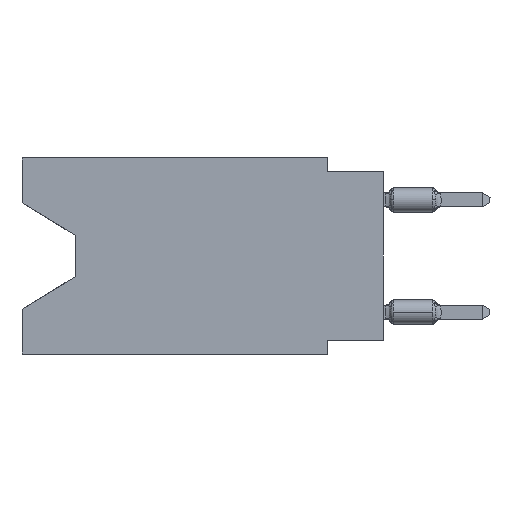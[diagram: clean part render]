
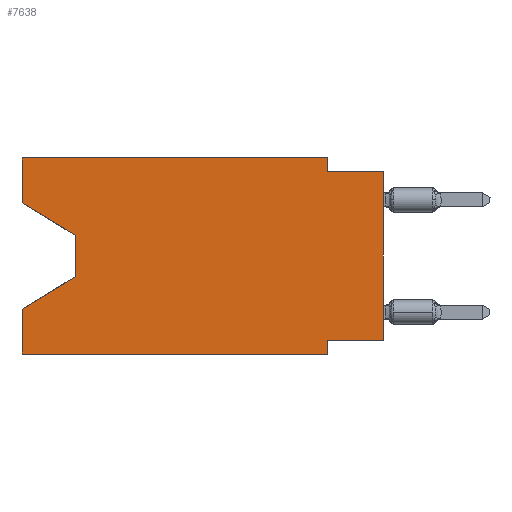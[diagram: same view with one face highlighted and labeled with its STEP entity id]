
A CAD part, left-side view. The second image highlights one B-rep face of the part: STEP entity #7638.
In plain terms, the highlighted planar face has unit normal (-1, 0, 0).
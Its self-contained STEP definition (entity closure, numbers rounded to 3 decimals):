
#333 = VECTOR ( 'NONE', #24219, 1000. ) ;
#567 = CARTESIAN_POINT ( 'NONE',  ( 0., 16.383, 0. ) ) ;
#601 = CARTESIAN_POINT ( 'NONE',  ( 0., 13.97, -5.385 ) ) ;
#702 = EDGE_CURVE ( 'NONE', #13876, #2454, #21498, .T. ) ;
#1024 = DIRECTION ( 'NONE',  ( 0., -1., 0. ) ) ;
#1044 = VECTOR ( 'NONE', #23749, 1000. ) ;
#1051 = CARTESIAN_POINT ( 'NONE',  ( 0., 16.383, 0. ) ) ;
#1136 = VECTOR ( 'NONE', #9603, 1000. ) ;
#1296 = VECTOR ( 'NONE', #15050, 1000. ) ;
#1582 = EDGE_LOOP ( 'NONE', ( #3260, #3955, #20768, #3757, #7621, #11592, #12425, #11807, #28553, #17022, #10541, #20219 ) ) ;
#2454 = VERTEX_POINT ( 'NONE', #13419 ) ;
#2486 = VECTOR ( 'NONE', #19190, 1000. ) ;
#2533 = EDGE_CURVE ( 'NONE', #17862, #22297, #10644, .T. ) ;
#2642 = VECTOR ( 'NONE', #14974, 1000. ) ;
#3260 = ORIENTED_EDGE ( 'NONE', *, *, #9465, .T. ) ;
#3692 = EDGE_CURVE ( 'NONE', #17862, #13538, #23213, .T. ) ;
#3741 = VECTOR ( 'NONE', #12759, 1000. ) ;
#3757 = ORIENTED_EDGE ( 'NONE', *, *, #12318, .F. ) ;
#3955 = ORIENTED_EDGE ( 'NONE', *, *, #20368, .T. ) ;
#4307 = EDGE_CURVE ( 'NONE', #2454, #22297, #23938, .T. ) ;
#4507 = LINE ( 'NONE', #23024, #11135 ) ;
#4675 = CARTESIAN_POINT ( 'NONE',  ( 0., 0., -8.255 ) ) ;
#4863 = VERTEX_POINT ( 'NONE', #23755 ) ;
#5017 = LINE ( 'NONE', #16282, #16054 ) ;
#5387 = VERTEX_POINT ( 'NONE', #29413 ) ;
#5941 = CARTESIAN_POINT ( 'NONE',  ( 0., 16.383, 0. ) ) ;
#7077 = LINE ( 'NONE', #12732, #1296 ) ;
#7621 = ORIENTED_EDGE ( 'NONE', *, *, #10113, .T. ) ;
#7638 = ADVANCED_FACE ( 'NONE', ( #10251 ), #17053, .F. ) ;
#8627 = VECTOR ( 'NONE', #15701, 1000. ) ;
#9268 = DIRECTION ( 'NONE',  ( 0., -0.855, -0.519 ) ) ;
#9465 = EDGE_CURVE ( 'NONE', #11706, #21772, #4507, .T. ) ;
#9603 = DIRECTION ( 'NONE',  ( 0., 1., 0. ) ) ;
#9775 = CARTESIAN_POINT ( 'NONE',  ( 0., 2.54, 0. ) ) ;
#10103 = DIRECTION ( 'NONE',  ( 1., 0., 0. ) ) ;
#10113 = EDGE_CURVE ( 'NONE', #15246, #10307, #7077, .T. ) ;
#10115 = CARTESIAN_POINT ( 'NONE',  ( 0., 2.54, 0. ) ) ;
#10251 = FACE_OUTER_BOUND ( 'NONE', #1582, .T. ) ;
#10307 = VERTEX_POINT ( 'NONE', #27705 ) ;
#10541 = ORIENTED_EDGE ( 'NONE', *, *, #26278, .F. ) ;
#10644 = LINE ( 'NONE', #17600, #13380 ) ;
#11135 = VECTOR ( 'NONE', #9268, 1000. ) ;
#11202 = EDGE_CURVE ( 'NONE', #11706, #5387, #24356, .T. ) ;
#11592 = ORIENTED_EDGE ( 'NONE', *, *, #20954, .F. ) ;
#11706 = VERTEX_POINT ( 'NONE', #29972 ) ;
#11807 = ORIENTED_EDGE ( 'NONE', *, *, #2533, .T. ) ;
#12318 = EDGE_CURVE ( 'NONE', #15246, #27703, #26377, .T. ) ;
#12425 = ORIENTED_EDGE ( 'NONE', *, *, #3692, .F. ) ;
#12732 = CARTESIAN_POINT ( 'NONE',  ( 0., 16.383, -8.89 ) ) ;
#12759 = DIRECTION ( 'NONE',  ( 0., 0., 1. ) ) ;
#13380 = VECTOR ( 'NONE', #27020, 1000. ) ;
#13419 = CARTESIAN_POINT ( 'NONE',  ( 0., 2.54, -0.635 ) ) ;
#13538 = VERTEX_POINT ( 'NONE', #24063 ) ;
#13876 = VERTEX_POINT ( 'NONE', #10115 ) ;
#14329 = CARTESIAN_POINT ( 'NONE',  ( 0., 16.383, 0. ) ) ;
#14974 = DIRECTION ( 'NONE',  ( 0., -1., 0. ) ) ;
#15050 = DIRECTION ( 'NONE',  ( 0., -1., 0. ) ) ;
#15246 = VERTEX_POINT ( 'NONE', #22180 ) ;
#15701 = DIRECTION ( 'NONE',  ( 0., 0., -1. ) ) ;
#16007 = LINE ( 'NONE', #20189, #8627 ) ;
#16054 = VECTOR ( 'NONE', #28176, 1000. ) ;
#16282 = CARTESIAN_POINT ( 'NONE',  ( 0., 2.54, -8.89 ) ) ;
#16676 = CARTESIAN_POINT ( 'NONE',  ( 0., 0., -0.635 ) ) ;
#16900 = DIRECTION ( 'NONE',  ( 0., 0., -1. ) ) ;
#17022 = ORIENTED_EDGE ( 'NONE', *, *, #702, .F. ) ;
#17053 = PLANE ( 'NONE',  #27322 ) ;
#17600 = CARTESIAN_POINT ( 'NONE',  ( 0., 0., 0. ) ) ;
#17862 = VERTEX_POINT ( 'NONE', #18491 ) ;
#18491 = CARTESIAN_POINT ( 'NONE',  ( 0., 0., -8.255 ) ) ;
#19190 = DIRECTION ( 'NONE',  ( 0., 0., -1. ) ) ;
#20189 = CARTESIAN_POINT ( 'NONE',  ( 0., 13.97, -3.505 ) ) ;
#20219 = ORIENTED_EDGE ( 'NONE', *, *, #11202, .F. ) ;
#20368 = EDGE_CURVE ( 'NONE', #21772, #4863, #16007, .T. ) ;
#20768 = ORIENTED_EDGE ( 'NONE', *, *, #28742, .T. ) ;
#20954 = EDGE_CURVE ( 'NONE', #13538, #10307, #5017, .T. ) ;
#21498 = LINE ( 'NONE', #9775, #2486 ) ;
#21772 = VERTEX_POINT ( 'NONE', #25930 ) ;
#22180 = CARTESIAN_POINT ( 'NONE',  ( 0., 16.383, -8.89 ) ) ;
#22297 = VERTEX_POINT ( 'NONE', #24459 ) ;
#23024 = CARTESIAN_POINT ( 'NONE',  ( 0., 16.383, -2.038 ) ) ;
#23213 = LINE ( 'NONE', #4675, #1136 ) ;
#23749 = DIRECTION ( 'NONE',  ( 0., 0.855, -0.519 ) ) ;
#23755 = CARTESIAN_POINT ( 'NONE',  ( 0., 13.97, -5.385 ) ) ;
#23938 = LINE ( 'NONE', #16676, #2642 ) ;
#24063 = CARTESIAN_POINT ( 'NONE',  ( 0., 2.54, -8.255 ) ) ;
#24086 = VECTOR ( 'NONE', #1024, 1000. ) ;
#24219 = DIRECTION ( 'NONE',  ( 0., 0., 1. ) ) ;
#24356 = LINE ( 'NONE', #1051, #3741 ) ;
#24459 = CARTESIAN_POINT ( 'NONE',  ( 0., 0., -0.635 ) ) ;
#25930 = CARTESIAN_POINT ( 'NONE',  ( 0., 13.97, -3.505 ) ) ;
#26055 = LINE ( 'NONE', #601, #1044 ) ;
#26278 = EDGE_CURVE ( 'NONE', #5387, #13876, #29726, .T. ) ;
#26377 = LINE ( 'NONE', #14329, #333 ) ;
#27020 = DIRECTION ( 'NONE',  ( 0., 0., 1. ) ) ;
#27322 = AXIS2_PLACEMENT_3D ( 'NONE', #567, #10103, #16900 ) ;
#27703 = VERTEX_POINT ( 'NONE', #29439 ) ;
#27705 = CARTESIAN_POINT ( 'NONE',  ( 0., 2.54, -8.89 ) ) ;
#28176 = DIRECTION ( 'NONE',  ( 0., 0., -1. ) ) ;
#28553 = ORIENTED_EDGE ( 'NONE', *, *, #4307, .F. ) ;
#28742 = EDGE_CURVE ( 'NONE', #4863, #27703, #26055, .T. ) ;
#29413 = CARTESIAN_POINT ( 'NONE',  ( 0., 16.383, 0. ) ) ;
#29439 = CARTESIAN_POINT ( 'NONE',  ( 0., 16.383, -6.852 ) ) ;
#29726 = LINE ( 'NONE', #5941, #24086 ) ;
#29972 = CARTESIAN_POINT ( 'NONE',  ( 0., 16.383, -2.038 ) ) ;
